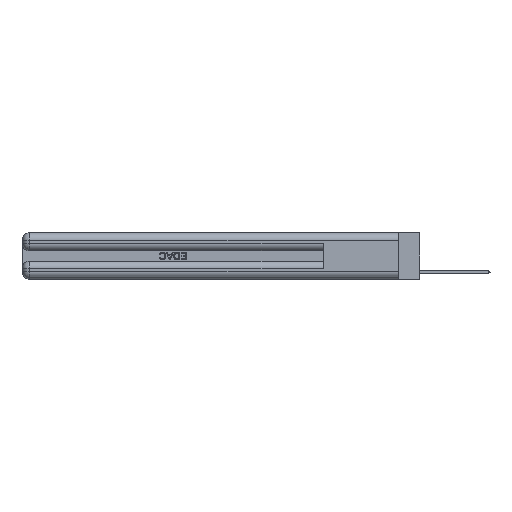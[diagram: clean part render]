
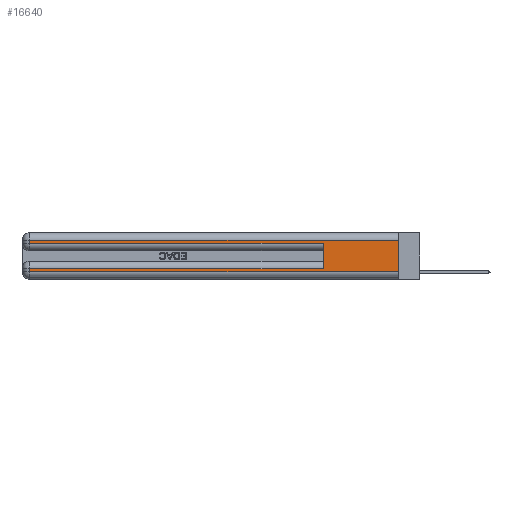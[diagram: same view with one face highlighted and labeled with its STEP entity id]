
A CAD part, left-side view. The second image highlights one B-rep face of the part: STEP entity #16640.
In plain terms, the highlighted planar face has unit normal (-1, 0, 0).
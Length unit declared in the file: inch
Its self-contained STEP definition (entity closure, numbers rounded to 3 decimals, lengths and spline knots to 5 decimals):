
#77 = CARTESIAN_POINT ( 'NONE',  ( 0., 0., 0.085 ) ) ;
#343 = CARTESIAN_POINT ( 'NONE',  ( 0., 0., 0.37 ) ) ;
#410 = VERTEX_POINT ( 'NONE', #12465 ) ;
#852 = VERTEX_POINT ( 'NONE', #29083 ) ;
#1310 = ORIENTED_EDGE ( 'NONE', *, *, #27387, .T. ) ;
#2048 = DIRECTION ( 'NONE',  ( 0., 0., -1. ) ) ;
#2098 = VECTOR ( 'NONE', #19260, 39.37008 ) ;
#2434 = EDGE_CURVE ( 'NONE', #852, #3681, #8227, .T. ) ;
#3403 = CARTESIAN_POINT ( 'NONE',  ( 0., 0., 0.06 ) ) ;
#3681 = VERTEX_POINT ( 'NONE', #3403 ) ;
#3856 = ORIENTED_EDGE ( 'NONE', *, *, #13277, .T. ) ;
#4140 = CARTESIAN_POINT ( 'NONE',  ( 0., 2.94, 0.37 ) ) ;
#5465 = LINE ( 'NONE', #7838, #32773 ) ;
#5557 = DIRECTION ( 'NONE',  ( 1., 0., 0. ) ) ;
#6333 = LINE ( 'NONE', #9452, #19331 ) ;
#6444 = LINE ( 'NONE', #77, #27492 ) ;
#6448 = EDGE_CURVE ( 'NONE', #410, #3681, #10936, .T. ) ;
#6765 = CARTESIAN_POINT ( 'NONE',  ( 0., 2.94, 0.085 ) ) ;
#7073 = CARTESIAN_POINT ( 'NONE',  ( 0., 0.6, 0.285 ) ) ;
#7838 = CARTESIAN_POINT ( 'NONE',  ( 0., 2.94, 0.37 ) ) ;
#8227 = LINE ( 'NONE', #343, #20418 ) ;
#8250 = AXIS2_PLACEMENT_3D ( 'NONE', #21672, #5557, #27071 ) ;
#8401 = ORIENTED_EDGE ( 'NONE', *, *, #2434, .F. ) ;
#9452 = CARTESIAN_POINT ( 'NONE',  ( 0., 0., 0.31 ) ) ;
#10936 = LINE ( 'NONE', #22958, #34435 ) ;
#11637 = ORIENTED_EDGE ( 'NONE', *, *, #17120, .F. ) ;
#12408 = EDGE_CURVE ( 'NONE', #26506, #24259, #5465, .T. ) ;
#12465 = CARTESIAN_POINT ( 'NONE',  ( 0., 2.94, 0.06 ) ) ;
#13277 = EDGE_CURVE ( 'NONE', #852, #26506, #6333, .T. ) ;
#13279 = CARTESIAN_POINT ( 'NONE',  ( 0., 2.94, 0.285 ) ) ;
#14435 = LINE ( 'NONE', #4140, #21535 ) ;
#15752 = CARTESIAN_POINT ( 'NONE',  ( 0., 0., 0.285 ) ) ;
#16241 = PLANE ( 'NONE',  #8250 ) ;
#16423 = DIRECTION ( 'NONE',  ( 0., 1., 0. ) ) ;
#16546 = CARTESIAN_POINT ( 'NONE',  ( 0., 0.6, 0.145 ) ) ;
#16640 = ADVANCED_FACE ( 'NONE', ( #19836 ), #16241, .F. ) ;
#17120 = EDGE_CURVE ( 'NONE', #26113, #25942, #34011, .T. ) ;
#19260 = DIRECTION ( 'NONE',  ( 0., 0., 1. ) ) ;
#19331 = VECTOR ( 'NONE', #31259, 39.37008 ) ;
#19836 = FACE_OUTER_BOUND ( 'NONE', #26801, .T. ) ;
#20418 = VECTOR ( 'NONE', #29954, 39.37008 ) ;
#21535 = VECTOR ( 'NONE', #33271, 39.37008 ) ;
#21672 = CARTESIAN_POINT ( 'NONE',  ( 0., 0., 0.37 ) ) ;
#22958 = CARTESIAN_POINT ( 'NONE',  ( 0., 0., 0.06 ) ) ;
#23528 = DIRECTION ( 'NONE',  ( 0., -1., 0. ) ) ;
#23857 = LINE ( 'NONE', #15752, #30143 ) ;
#24259 = VERTEX_POINT ( 'NONE', #13279 ) ;
#25591 = ORIENTED_EDGE ( 'NONE', *, *, #26594, .T. ) ;
#25942 = VERTEX_POINT ( 'NONE', #7073 ) ;
#26006 = DIRECTION ( 'NONE',  ( 0., -1., 0. ) ) ;
#26113 = VERTEX_POINT ( 'NONE', #31564 ) ;
#26506 = VERTEX_POINT ( 'NONE', #27138 ) ;
#26594 = EDGE_CURVE ( 'NONE', #26113, #29542, #6444, .T. ) ;
#26801 = EDGE_LOOP ( 'NONE', ( #8401, #3856, #31747, #31781, #11637, #25591, #1310, #30993 ) ) ;
#27071 = DIRECTION ( 'NONE',  ( 0., 0., -1. ) ) ;
#27138 = CARTESIAN_POINT ( 'NONE',  ( 0., 2.94, 0.31 ) ) ;
#27387 = EDGE_CURVE ( 'NONE', #29542, #410, #14435, .T. ) ;
#27492 = VECTOR ( 'NONE', #16423, 39.37008 ) ;
#29083 = CARTESIAN_POINT ( 'NONE',  ( 0., 0., 0.31 ) ) ;
#29542 = VERTEX_POINT ( 'NONE', #6765 ) ;
#29954 = DIRECTION ( 'NONE',  ( 0., 0., -1. ) ) ;
#30143 = VECTOR ( 'NONE', #23528, 39.37008 ) ;
#30993 = ORIENTED_EDGE ( 'NONE', *, *, #6448, .T. ) ;
#31259 = DIRECTION ( 'NONE',  ( 0., 1., 0. ) ) ;
#31564 = CARTESIAN_POINT ( 'NONE',  ( 0., 0.6, 0.085 ) ) ;
#31747 = ORIENTED_EDGE ( 'NONE', *, *, #12408, .T. ) ;
#31781 = ORIENTED_EDGE ( 'NONE', *, *, #34140, .T. ) ;
#32773 = VECTOR ( 'NONE', #2048, 39.37008 ) ;
#33271 = DIRECTION ( 'NONE',  ( 0., 0., -1. ) ) ;
#34011 = LINE ( 'NONE', #16546, #2098 ) ;
#34140 = EDGE_CURVE ( 'NONE', #24259, #25942, #23857, .T. ) ;
#34435 = VECTOR ( 'NONE', #26006, 39.37008 ) ;
